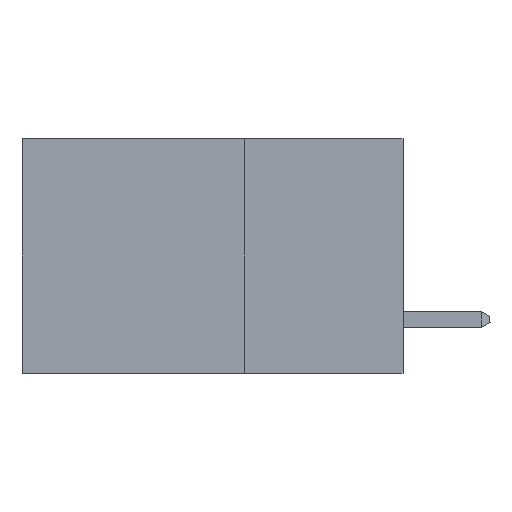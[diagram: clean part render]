
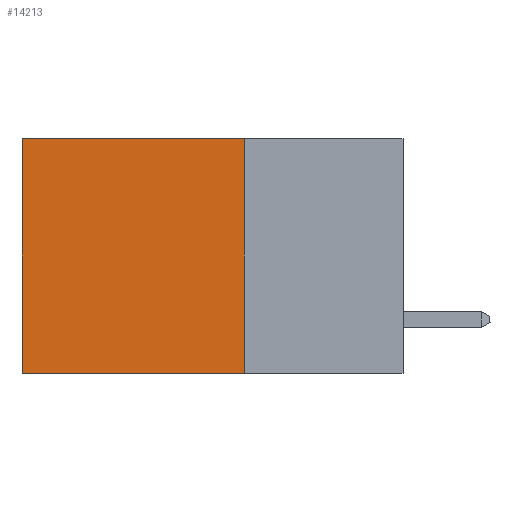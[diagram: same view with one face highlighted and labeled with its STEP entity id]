
A CAD part, left-side view. The second image highlights one B-rep face of the part: STEP entity #14213.
In plain terms, the highlighted planar face has unit normal (-1, 0, 0).
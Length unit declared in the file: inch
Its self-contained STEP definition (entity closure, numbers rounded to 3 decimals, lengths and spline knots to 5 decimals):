
#232 = EDGE_CURVE ( 'NONE', #16558, #4303, #8899, .T. ) ;
#428 = PLANE ( 'NONE',  #17006 ) ;
#2898 = ORIENTED_EDGE ( 'NONE', *, *, #232, .T. ) ;
#3144 = VECTOR ( 'NONE', #13619, 39.37008 ) ;
#3215 = DIRECTION ( 'NONE',  ( 0., 0., -1. ) ) ;
#4006 = CARTESIAN_POINT ( 'NONE',  ( 0.2875, 0.6, 0. ) ) ;
#4062 = VERTEX_POINT ( 'NONE', #15943 ) ;
#4303 = VERTEX_POINT ( 'NONE', #7208 ) ;
#4778 = DIRECTION ( 'NONE',  ( 1., 0., 0. ) ) ;
#5312 = DIRECTION ( 'NONE',  ( 0., 1., 0. ) ) ;
#6845 = DIRECTION ( 'NONE',  ( 0., 0., -1. ) ) ;
#7208 = CARTESIAN_POINT ( 'NONE',  ( 0.2875, 0.6, -0.37 ) ) ;
#7595 = EDGE_CURVE ( 'NONE', #11117, #4062, #7764, .T. ) ;
#7764 = LINE ( 'NONE', #17645, #11029 ) ;
#8346 = CARTESIAN_POINT ( 'NONE',  ( 0.2875, 0.25, -0.37 ) ) ;
#8899 = LINE ( 'NONE', #4006, #3144 ) ;
#9430 = CARTESIAN_POINT ( 'NONE',  ( 0.2875, 0.25, 0. ) ) ;
#9787 = VECTOR ( 'NONE', #5312, 39.37008 ) ;
#11029 = VECTOR ( 'NONE', #6845, 39.37008 ) ;
#11117 = VERTEX_POINT ( 'NONE', #17731 ) ;
#12565 = EDGE_LOOP ( 'NONE', ( #2898, #14560, #13955, #14205 ) ) ;
#12789 = VECTOR ( 'NONE', #16493, 39.37008 ) ;
#13209 = FACE_OUTER_BOUND ( 'NONE', #12565, .T. ) ;
#13395 = LINE ( 'NONE', #9430, #9787 ) ;
#13619 = DIRECTION ( 'NONE',  ( 0., 0., -1. ) ) ;
#13955 = ORIENTED_EDGE ( 'NONE', *, *, #7595, .F. ) ;
#14205 = ORIENTED_EDGE ( 'NONE', *, *, #17955, .T. ) ;
#14213 = ADVANCED_FACE ( 'NONE', ( #13209 ), #428, .F. ) ;
#14402 = CARTESIAN_POINT ( 'NONE',  ( 0.2875, 0.6, 0. ) ) ;
#14560 = ORIENTED_EDGE ( 'NONE', *, *, #17346, .F. ) ;
#15835 = CARTESIAN_POINT ( 'NONE',  ( 0.2875, 0.25, 0. ) ) ;
#15943 = CARTESIAN_POINT ( 'NONE',  ( 0.2875, 0.25, -0.37 ) ) ;
#16493 = DIRECTION ( 'NONE',  ( 0., 1., 0. ) ) ;
#16500 = LINE ( 'NONE', #8346, #12789 ) ;
#16558 = VERTEX_POINT ( 'NONE', #14402 ) ;
#17006 = AXIS2_PLACEMENT_3D ( 'NONE', #15835, #4778, #3215 ) ;
#17346 = EDGE_CURVE ( 'NONE', #4062, #4303, #16500, .T. ) ;
#17645 = CARTESIAN_POINT ( 'NONE',  ( 0.2875, 0.25, 0. ) ) ;
#17731 = CARTESIAN_POINT ( 'NONE',  ( 0.2875, 0.25, 0. ) ) ;
#17955 = EDGE_CURVE ( 'NONE', #11117, #16558, #13395, .T. ) ;
